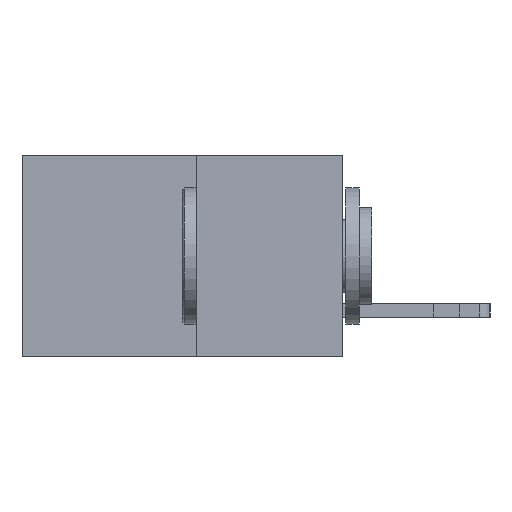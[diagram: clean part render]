
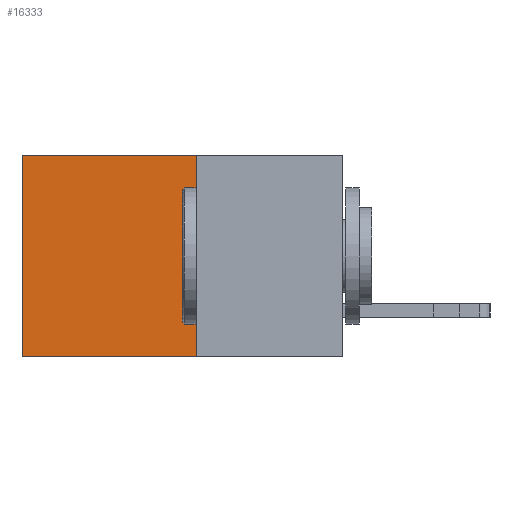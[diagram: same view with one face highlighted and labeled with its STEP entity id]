
A CAD part, left-side view. The second image highlights one B-rep face of the part: STEP entity #16333.
In plain terms, the highlighted planar face has unit normal (-1, 0, 0).
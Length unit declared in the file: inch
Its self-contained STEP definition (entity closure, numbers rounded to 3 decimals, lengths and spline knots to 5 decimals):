
#887 = EDGE_CURVE ( 'NONE', #3228, #1539, #19038, .T. ) ;
#1373 = CARTESIAN_POINT ( 'NONE',  ( 0.277, 0.27, 0. ) ) ;
#1539 = VERTEX_POINT ( 'NONE', #17879 ) ;
#1848 = EDGE_CURVE ( 'NONE', #13827, #16270, #15926, .T. ) ;
#1856 = DIRECTION ( 'NONE',  ( 1., 0., 0. ) ) ;
#2932 = EDGE_LOOP ( 'NONE', ( #3246, #10600, #16499, #16669 ) ) ;
#3228 = VERTEX_POINT ( 'NONE', #16708 ) ;
#3246 = ORIENTED_EDGE ( 'NONE', *, *, #7544, .T. ) ;
#3331 = CARTESIAN_POINT ( 'NONE',  ( 0.277, 0.27, -0.37 ) ) ;
#4174 = DIRECTION ( 'NONE',  ( 0., 1., 0. ) ) ;
#5088 = CARTESIAN_POINT ( 'NONE',  ( 0.277, 0.59, -0.37 ) ) ;
#5769 = CARTESIAN_POINT ( 'NONE',  ( 0.277, 0.27, -0.37 ) ) ;
#6586 = DIRECTION ( 'NONE',  ( 0., 0., -1. ) ) ;
#7034 = CARTESIAN_POINT ( 'NONE',  ( 0.277, 0.27, 0. ) ) ;
#7308 = DIRECTION ( 'NONE',  ( 0., 1., 0. ) ) ;
#7544 = EDGE_CURVE ( 'NONE', #16270, #1539, #10506, .T. ) ;
#8093 = CARTESIAN_POINT ( 'NONE',  ( 0.277, 0.27, -0.37 ) ) ;
#8116 = VECTOR ( 'NONE', #7308, 39.37008 ) ;
#8400 = VECTOR ( 'NONE', #11015, 39.37008 ) ;
#10020 = VECTOR ( 'NONE', #6586, 39.37008 ) ;
#10506 = LINE ( 'NONE', #5088, #10020 ) ;
#10600 = ORIENTED_EDGE ( 'NONE', *, *, #887, .F. ) ;
#11015 = DIRECTION ( 'NONE',  ( 0., 0., -1. ) ) ;
#12396 = AXIS2_PLACEMENT_3D ( 'NONE', #8093, #1856, #12650 ) ;
#12584 = PLANE ( 'NONE',  #12396 ) ;
#12650 = DIRECTION ( 'NONE',  ( 0., 0., -1. ) ) ;
#12872 = LINE ( 'NONE', #3331, #8400 ) ;
#13827 = VERTEX_POINT ( 'NONE', #1373 ) ;
#13837 = FACE_OUTER_BOUND ( 'NONE', #2932, .T. ) ;
#15926 = LINE ( 'NONE', #7034, #8116 ) ;
#16270 = VERTEX_POINT ( 'NONE', #18128 ) ;
#16333 = ADVANCED_FACE ( 'NONE', ( #13837 ), #12584, .F. ) ;
#16499 = ORIENTED_EDGE ( 'NONE', *, *, #16824, .F. ) ;
#16669 = ORIENTED_EDGE ( 'NONE', *, *, #1848, .T. ) ;
#16708 = CARTESIAN_POINT ( 'NONE',  ( 0.277, 0.27, -0.37 ) ) ;
#16824 = EDGE_CURVE ( 'NONE', #13827, #3228, #12872, .T. ) ;
#17879 = CARTESIAN_POINT ( 'NONE',  ( 0.277, 0.59, -0.37 ) ) ;
#18128 = CARTESIAN_POINT ( 'NONE',  ( 0.277, 0.59, 0. ) ) ;
#18149 = VECTOR ( 'NONE', #4174, 39.37008 ) ;
#19038 = LINE ( 'NONE', #5769, #18149 ) ;
